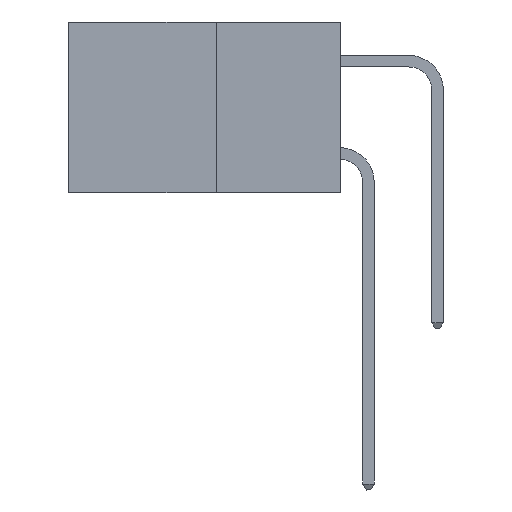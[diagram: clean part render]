
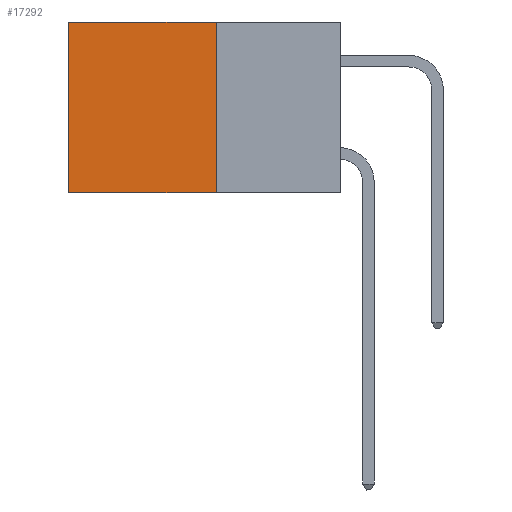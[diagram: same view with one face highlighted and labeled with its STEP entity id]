
A CAD part, left-side view. The second image highlights one B-rep face of the part: STEP entity #17292.
In plain terms, the highlighted planar face has unit normal (-1, 0, 0).
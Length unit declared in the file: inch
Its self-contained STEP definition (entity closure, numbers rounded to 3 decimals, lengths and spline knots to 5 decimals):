
#1621 = EDGE_CURVE ( 'NONE', #22160, #25484, #10799, .T. ) ;
#1685 = CARTESIAN_POINT ( 'NONE',  ( 0.277, 0.59, 0. ) ) ;
#2280 = VECTOR ( 'NONE', #7934, 39.37008 ) ;
#2658 = DIRECTION ( 'NONE',  ( 0., 0., -1. ) ) ;
#3306 = CARTESIAN_POINT ( 'NONE',  ( 0.277, 0.59, -0.37 ) ) ;
#4106 = FACE_OUTER_BOUND ( 'NONE', #8498, .T. ) ;
#4380 = CARTESIAN_POINT ( 'NONE',  ( 0.277, 0.27, -0.37 ) ) ;
#4415 = EDGE_CURVE ( 'NONE', #20513, #8707, #10117, .T. ) ;
#5469 = DIRECTION ( 'NONE',  ( 0., 1., 0. ) ) ;
#5668 = CARTESIAN_POINT ( 'NONE',  ( 0.277, 0.59, -0.37 ) ) ;
#6355 = EDGE_CURVE ( 'NONE', #20513, #22160, #8194, .T. ) ;
#6359 = EDGE_CURVE ( 'NONE', #8707, #25484, #13428, .T. ) ;
#6401 = DIRECTION ( 'NONE',  ( 0., 0., -1. ) ) ;
#7934 = DIRECTION ( 'NONE',  ( 0., 1., 0. ) ) ;
#8194 = LINE ( 'NONE', #10340, #18102 ) ;
#8498 = EDGE_LOOP ( 'NONE', ( #21645, #9411, #20103, #15422 ) ) ;
#8707 = VERTEX_POINT ( 'NONE', #23749 ) ;
#9411 = ORIENTED_EDGE ( 'NONE', *, *, #6359, .F. ) ;
#10117 = LINE ( 'NONE', #21848, #16645 ) ;
#10340 = CARTESIAN_POINT ( 'NONE',  ( 0.277, 0.27, 0. ) ) ;
#10516 = CARTESIAN_POINT ( 'NONE',  ( 0.277, 0.27, -0.37 ) ) ;
#10799 = LINE ( 'NONE', #3306, #25374 ) ;
#12377 = DIRECTION ( 'NONE',  ( 0., 0., -1. ) ) ;
#13428 = LINE ( 'NONE', #10516, #2280 ) ;
#13713 = CARTESIAN_POINT ( 'NONE',  ( 0.277, 0.27, 0. ) ) ;
#15422 = ORIENTED_EDGE ( 'NONE', *, *, #6355, .T. ) ;
#16225 = PLANE ( 'NONE',  #20863 ) ;
#16645 = VECTOR ( 'NONE', #12377, 39.37008 ) ;
#17292 = ADVANCED_FACE ( 'NONE', ( #4106 ), #16225, .F. ) ;
#18102 = VECTOR ( 'NONE', #5469, 39.37008 ) ;
#18219 = DIRECTION ( 'NONE',  ( 1., 0., 0. ) ) ;
#20103 = ORIENTED_EDGE ( 'NONE', *, *, #4415, .F. ) ;
#20513 = VERTEX_POINT ( 'NONE', #13713 ) ;
#20863 = AXIS2_PLACEMENT_3D ( 'NONE', #4380, #18219, #6401 ) ;
#21645 = ORIENTED_EDGE ( 'NONE', *, *, #1621, .T. ) ;
#21848 = CARTESIAN_POINT ( 'NONE',  ( 0.277, 0.27, -0.37 ) ) ;
#22160 = VERTEX_POINT ( 'NONE', #1685 ) ;
#23749 = CARTESIAN_POINT ( 'NONE',  ( 0.277, 0.27, -0.37 ) ) ;
#25374 = VECTOR ( 'NONE', #2658, 39.37008 ) ;
#25484 = VERTEX_POINT ( 'NONE', #5668 ) ;
